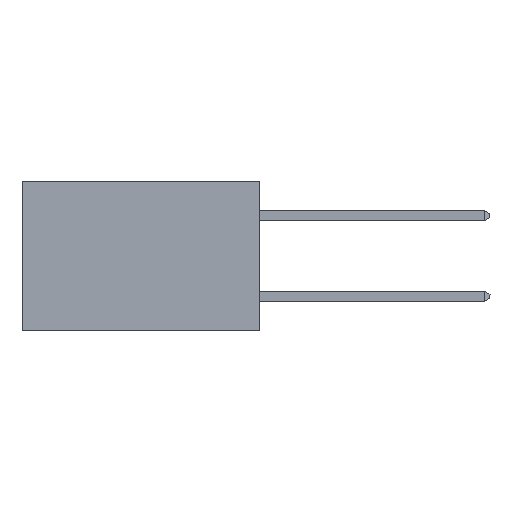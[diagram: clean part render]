
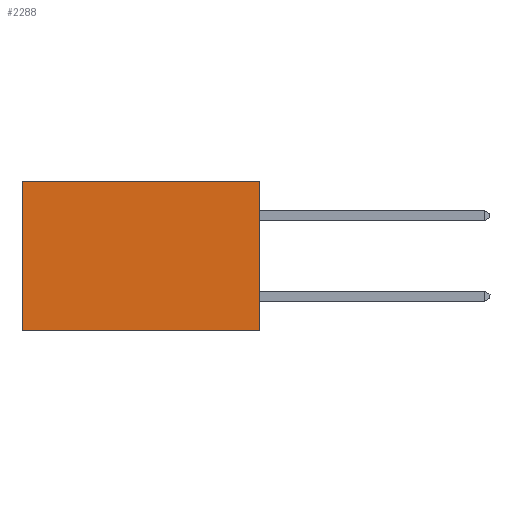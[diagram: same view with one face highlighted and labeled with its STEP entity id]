
A CAD part, left-side view. The second image highlights one B-rep face of the part: STEP entity #2288.
In plain terms, the highlighted planar face has unit normal (-1, 0, 0).
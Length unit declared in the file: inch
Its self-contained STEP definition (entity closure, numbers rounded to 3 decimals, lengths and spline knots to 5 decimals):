
#127 = VECTOR ( 'NONE', #2062, 39.37008 ) ;
#294 = ORIENTED_EDGE ( 'NONE', *, *, #3707, .T. ) ;
#365 = EDGE_CURVE ( 'NONE', #3082, #7520, #7002, .T. ) ;
#894 = EDGE_CURVE ( 'NONE', #4666, #7520, #4508, .T. ) ;
#1110 = EDGE_LOOP ( 'NONE', ( #2095, #8721, #1913, #294 ) ) ;
#1722 = VECTOR ( 'NONE', #3283, 39.37008 ) ;
#1913 = ORIENTED_EDGE ( 'NONE', *, *, #4019, .F. ) ;
#2062 = DIRECTION ( 'NONE',  ( 0., 1., 0. ) ) ;
#2084 = LINE ( 'NONE', #9353, #12004 ) ;
#2095 = ORIENTED_EDGE ( 'NONE', *, *, #365, .T. ) ;
#2255 = CARTESIAN_POINT ( 'NONE',  ( 0.277, 0., 0. ) ) ;
#2288 = ADVANCED_FACE ( 'NONE', ( #6789 ), #8310, .F. ) ;
#2739 = CARTESIAN_POINT ( 'NONE',  ( 0.277, 0.59, 0. ) ) ;
#3082 = VERTEX_POINT ( 'NONE', #2739 ) ;
#3283 = DIRECTION ( 'NONE',  ( 0., 1., 0. ) ) ;
#3707 = EDGE_CURVE ( 'NONE', #9139, #3082, #8269, .T. ) ;
#4019 = EDGE_CURVE ( 'NONE', #9139, #4666, #2084, .T. ) ;
#4092 = DIRECTION ( 'NONE',  ( 0., 0., -1. ) ) ;
#4508 = LINE ( 'NONE', #11526, #1722 ) ;
#4666 = VERTEX_POINT ( 'NONE', #8937 ) ;
#5109 = DIRECTION ( 'NONE',  ( 1., 0., 0. ) ) ;
#5381 = CARTESIAN_POINT ( 'NONE',  ( 0.277, 0.59, -0.37 ) ) ;
#6789 = FACE_OUTER_BOUND ( 'NONE', #1110, .T. ) ;
#6849 = AXIS2_PLACEMENT_3D ( 'NONE', #8651, #5109, #4092 ) ;
#7002 = LINE ( 'NONE', #11675, #11840 ) ;
#7520 = VERTEX_POINT ( 'NONE', #5381 ) ;
#7713 = DIRECTION ( 'NONE',  ( 0., 0., -1. ) ) ;
#8269 = LINE ( 'NONE', #2255, #127 ) ;
#8310 = PLANE ( 'NONE',  #6849 ) ;
#8651 = CARTESIAN_POINT ( 'NONE',  ( 0.277, 0., -0.37 ) ) ;
#8721 = ORIENTED_EDGE ( 'NONE', *, *, #894, .F. ) ;
#8741 = CARTESIAN_POINT ( 'NONE',  ( 0.277, 0., 0. ) ) ;
#8937 = CARTESIAN_POINT ( 'NONE',  ( 0.277, 0., -0.37 ) ) ;
#9139 = VERTEX_POINT ( 'NONE', #8741 ) ;
#9353 = CARTESIAN_POINT ( 'NONE',  ( 0.277, 0., -0.37 ) ) ;
#11526 = CARTESIAN_POINT ( 'NONE',  ( 0.277, 0., -0.37 ) ) ;
#11609 = DIRECTION ( 'NONE',  ( 0., 0., -1. ) ) ;
#11675 = CARTESIAN_POINT ( 'NONE',  ( 0.277, 0.59, -0.37 ) ) ;
#11840 = VECTOR ( 'NONE', #11609, 39.37008 ) ;
#12004 = VECTOR ( 'NONE', #7713, 39.37008 ) ;
